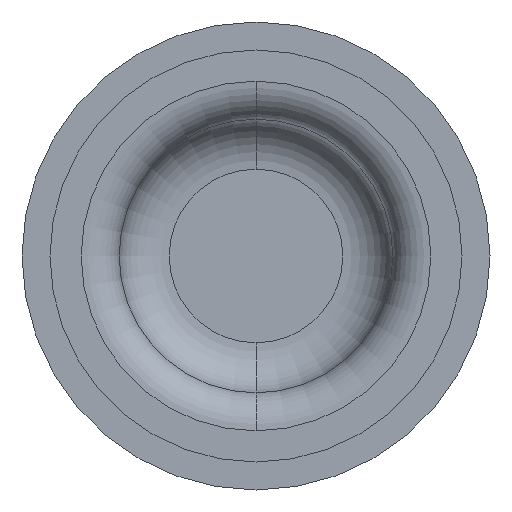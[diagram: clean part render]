
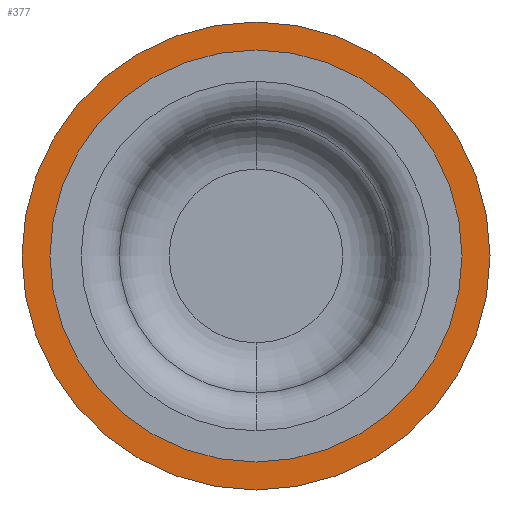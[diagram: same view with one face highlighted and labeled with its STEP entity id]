
A CAD part, front view. The second image highlights one B-rep face of the part: STEP entity #377.
In plain terms, the highlighted planar face has unit normal (0, -1, 0).
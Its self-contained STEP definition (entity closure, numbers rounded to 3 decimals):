
#21 = DIRECTION ( 'NONE',  ( 1., 0., 0. ) ) ;
#41 = EDGE_LOOP ( 'NONE', ( #624, #463 ) ) ;
#55 = CARTESIAN_POINT ( 'NONE',  ( 5.95, -36.722, 0. ) ) ;
#97 = VERTEX_POINT ( 'NONE', #368 ) ;
#117 = DIRECTION ( 'NONE',  ( -1., 0., 0. ) ) ;
#119 = DIRECTION ( 'NONE',  ( 0., 1., 0. ) ) ;
#122 = CARTESIAN_POINT ( 'NONE',  ( 0., -36.722, 0. ) ) ;
#140 = DIRECTION ( 'NONE',  ( 1., 0., 0. ) ) ;
#146 = VERTEX_POINT ( 'NONE', #346 ) ;
#177 = CIRCLE ( 'NONE', #644, 5.95 ) ;
#217 = DIRECTION ( 'NONE',  ( 0., 1., 0. ) ) ;
#223 = CARTESIAN_POINT ( 'NONE',  ( 0., -36.722, 0. ) ) ;
#230 = AXIS2_PLACEMENT_3D ( 'NONE', #618, #610, #607 ) ;
#295 = DIRECTION ( 'NONE',  ( 0., 0., -1. ) ) ;
#299 = EDGE_CURVE ( 'NONE', #146, #591, #517, .T. ) ;
#302 = DIRECTION ( 'NONE',  ( 0., -1., 0. ) ) ;
#310 = FACE_OUTER_BOUND ( 'NONE', #41, .T. ) ;
#314 = PLANE ( 'NONE',  #647 ) ;
#343 = EDGE_CURVE ( 'NONE', #591, #146, #500, .T. ) ;
#346 = CARTESIAN_POINT ( 'NONE',  ( 5.239, -36.722, 0. ) ) ;
#368 = CARTESIAN_POINT ( 'NONE',  ( -5.95, -36.722, 0. ) ) ;
#377 = ADVANCED_FACE ( 'NONE', ( #310, #627 ), #314, .T. ) ;
#383 = EDGE_CURVE ( 'NONE', #413, #97, #177, .T. ) ;
#413 = VERTEX_POINT ( 'NONE', #55 ) ;
#417 = EDGE_CURVE ( 'NONE', #97, #413, #626, .T. ) ;
#463 = ORIENTED_EDGE ( 'NONE', *, *, #383, .F. ) ;
#478 = AXIS2_PLACEMENT_3D ( 'NONE', #122, #119, #117 ) ;
#494 = CARTESIAN_POINT ( 'NONE',  ( -5.239, -36.722, 0. ) ) ;
#500 = CIRCLE ( 'NONE', #230, 5.239 ) ;
#517 = CIRCLE ( 'NONE', #478, 5.239 ) ;
#521 = ORIENTED_EDGE ( 'NONE', *, *, #299, .T. ) ;
#543 = CARTESIAN_POINT ( 'NONE',  ( 0., -36.722, 0. ) ) ;
#553 = ORIENTED_EDGE ( 'NONE', *, *, #343, .T. ) ;
#557 = CARTESIAN_POINT ( 'NONE',  ( -4.187, -36.722, 0. ) ) ;
#563 = AXIS2_PLACEMENT_3D ( 'NONE', #543, #576, #21 ) ;
#572 = EDGE_LOOP ( 'NONE', ( #553, #521 ) ) ;
#576 = DIRECTION ( 'NONE',  ( 0., 1., 0. ) ) ;
#591 = VERTEX_POINT ( 'NONE', #494 ) ;
#607 = DIRECTION ( 'NONE',  ( -1., 0., 0. ) ) ;
#610 = DIRECTION ( 'NONE',  ( 0., 1., 0. ) ) ;
#618 = CARTESIAN_POINT ( 'NONE',  ( 0., -36.722, 0. ) ) ;
#624 = ORIENTED_EDGE ( 'NONE', *, *, #417, .F. ) ;
#626 = CIRCLE ( 'NONE', #563, 5.95 ) ;
#627 = FACE_BOUND ( 'NONE', #572, .T. ) ;
#644 = AXIS2_PLACEMENT_3D ( 'NONE', #223, #217, #140 ) ;
#647 = AXIS2_PLACEMENT_3D ( 'NONE', #557, #302, #295 ) ;
